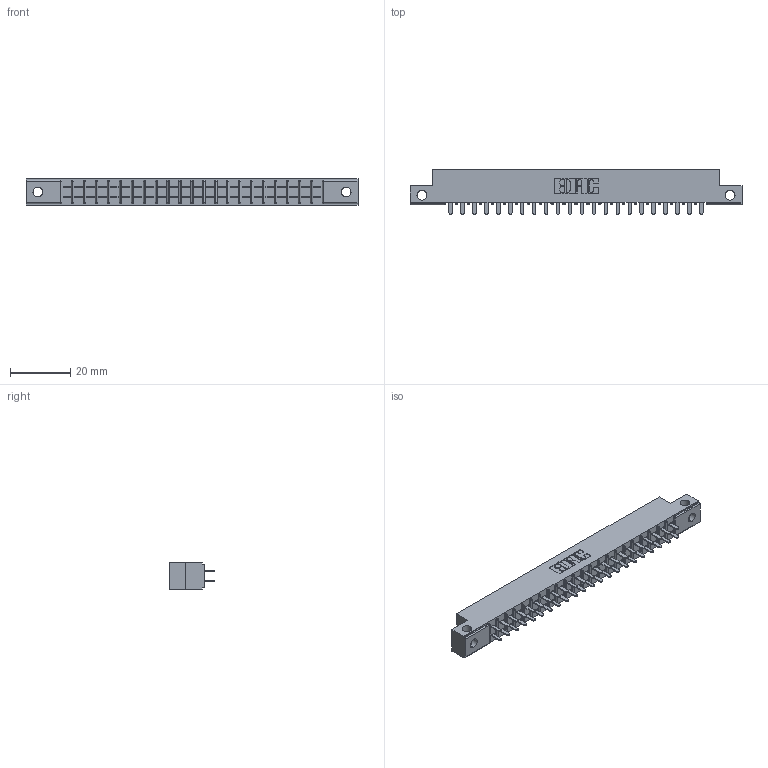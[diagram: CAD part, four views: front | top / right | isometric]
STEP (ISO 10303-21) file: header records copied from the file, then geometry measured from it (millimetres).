
FILE_DESCRIPTION (( 'STEP AP203' ), '1' );
FILE_NAME ('305-044-521-512.STEP', '2020-09-19T22:17:53', ( '' ), ( '' ), 'SwSTEP 2.0', 'SolidWorks 2020', '' );
FILE_SCHEMA (( 'CONFIG_CONTROL_DESIGN' ));
Length unit declared in the file: inch
Products named in the file (3): 305-044-521-512; 305 Part_.128 Dia; 305-290-001_521
Assembly tree (45 placements, depth 2):
  305-044-521-512
    305 Part_.128 Dia
    305-290-001_521  x44
Bounding box: 110.19 x 14.86 x 8.71 mm (x, y, z)
Volume: 6426.5 mm3; surface area: 12631.7 mm2
Topology: 45 solids, 45 shells, 2152 faces, 6138 edges, 3968 vertices
Faces by surface type: plane 1256, cylinder 808, sphere 88
Entity records: 26541 total; most frequent: CARTESIAN_POINT 4440, ORIENTED_EDGE 4360, DIRECTION 4250, EDGE_CURVE 2180, VECTOR 1726, LINE 1726, VERTEX_POINT 1388, AXIS2_PLACEMENT_3D 1262
